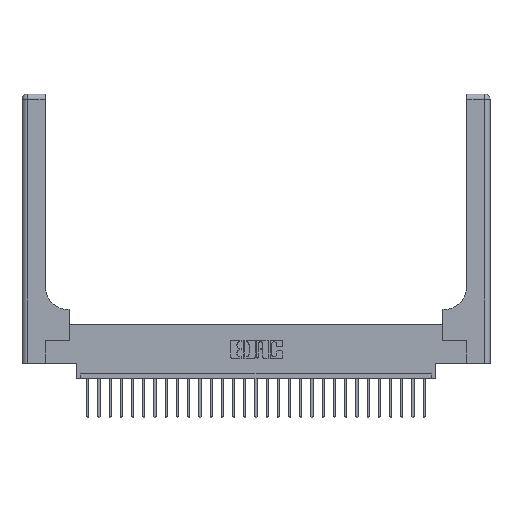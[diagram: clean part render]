
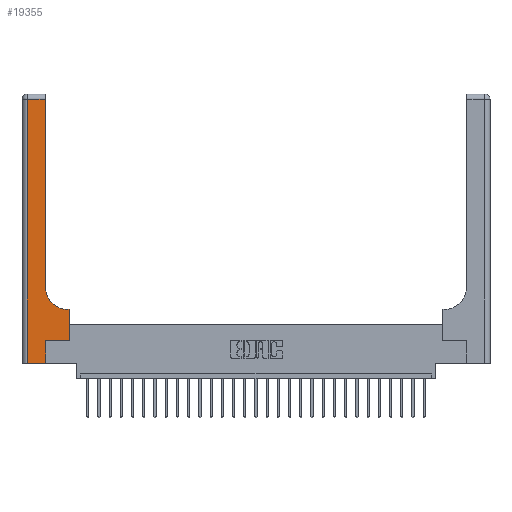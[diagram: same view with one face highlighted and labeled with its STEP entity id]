
A CAD part, top view. The second image highlights one B-rep face of the part: STEP entity #19355.
In plain terms, the highlighted planar face has unit normal (0, 0, 1).
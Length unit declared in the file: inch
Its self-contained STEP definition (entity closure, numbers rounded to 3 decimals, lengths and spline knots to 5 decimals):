
#160 = CARTESIAN_POINT ( 'NONE',  ( 0.06, 3., 0.37 ) ) ;
#386 = DIRECTION ( 'NONE',  ( 1., 0., 0. ) ) ;
#827 = CARTESIAN_POINT ( 'NONE',  ( 0.265, 0.25, 0.37 ) ) ;
#878 = CARTESIAN_POINT ( 'NONE',  ( 0., 0., 0.37 ) ) ;
#897 = EDGE_CURVE ( 'NONE', #14503, #10688, #25586, .T. ) ;
#1020 = PLANE ( 'NONE',  #8135 ) ;
#1361 = EDGE_CURVE ( 'NONE', #11129, #23837, #13041, .T. ) ;
#1598 = LINE ( 'NONE', #22780, #13895 ) ;
#1727 = EDGE_CURVE ( 'NONE', #13313, #22823, #15457, .T. ) ;
#2290 = CARTESIAN_POINT ( 'NONE',  ( 0.265, 0., 0.37 ) ) ;
#2490 = ORIENTED_EDGE ( 'NONE', *, *, #13686, .T. ) ;
#2798 = LINE ( 'NONE', #878, #13047 ) ;
#3026 = CARTESIAN_POINT ( 'NONE',  ( 0., 3., 0.37 ) ) ;
#3300 = VERTEX_POINT ( 'NONE', #10138 ) ;
#4204 = DIRECTION ( 'NONE',  ( 0., 1., 0. ) ) ;
#4282 = DIRECTION ( 'NONE',  ( 0., 1., 0. ) ) ;
#4557 = CARTESIAN_POINT ( 'NONE',  ( 0.51, 0.85, 0.37 ) ) ;
#4723 = DIRECTION ( 'NONE',  ( -1., 0., 0. ) ) ;
#4737 = ORIENTED_EDGE ( 'NONE', *, *, #11820, .T. ) ;
#5027 = DIRECTION ( 'NONE',  ( 0., 0., -1. ) ) ;
#5046 = LINE ( 'NONE', #19664, #20202 ) ;
#6188 = DIRECTION ( 'NONE',  ( 0., -1., 0. ) ) ;
#6428 = CARTESIAN_POINT ( 'NONE',  ( 0.528, 0.25, 0.37 ) ) ;
#6614 = AXIS2_PLACEMENT_3D ( 'NONE', #4557, #14737, #386 ) ;
#6826 = CARTESIAN_POINT ( 'NONE',  ( 0.528, 0.6, 0.37 ) ) ;
#6858 = VECTOR ( 'NONE', #12193, 39.37008 ) ;
#8135 = AXIS2_PLACEMENT_3D ( 'NONE', #3026, #5027, #19159 ) ;
#8582 = EDGE_LOOP ( 'NONE', ( #12353, #25006, #9893, #16631, #10606, #4737, #22381, #2490, #20142 ) ) ;
#8651 = VECTOR ( 'NONE', #4723, 39.37008 ) ;
#9507 = VECTOR ( 'NONE', #6188, 39.37008 ) ;
#9630 = EDGE_CURVE ( 'NONE', #23837, #3300, #1598, .T. ) ;
#9893 = ORIENTED_EDGE ( 'NONE', *, *, #897, .T. ) ;
#10138 = CARTESIAN_POINT ( 'NONE',  ( 0.26, 2.94, 0.37 ) ) ;
#10338 = CARTESIAN_POINT ( 'NONE',  ( 0.265, 0.25, 0.37 ) ) ;
#10366 = EDGE_CURVE ( 'NONE', #3300, #14503, #5046, .T. ) ;
#10606 = ORIENTED_EDGE ( 'NONE', *, *, #1727, .T. ) ;
#10688 = VERTEX_POINT ( 'NONE', #22925 ) ;
#11129 = VERTEX_POINT ( 'NONE', #23139 ) ;
#11820 = EDGE_CURVE ( 'NONE', #22823, #21023, #24253, .T. ) ;
#12193 = DIRECTION ( 'NONE',  ( 1., 0., 0. ) ) ;
#12239 = CARTESIAN_POINT ( 'NONE',  ( 0.06, 2.94, 0.37 ) ) ;
#12301 = EDGE_CURVE ( 'NONE', #21023, #16313, #16001, .T. ) ;
#12353 = ORIENTED_EDGE ( 'NONE', *, *, #9630, .T. ) ;
#13041 = CIRCLE ( 'NONE', #6614, 0.25 ) ;
#13047 = VECTOR ( 'NONE', #18924, 39.37008 ) ;
#13313 = VERTEX_POINT ( 'NONE', #20820 ) ;
#13686 = EDGE_CURVE ( 'NONE', #16313, #11129, #18451, .T. ) ;
#13774 = DIRECTION ( 'NONE',  ( -1., 0., 0. ) ) ;
#13895 = VECTOR ( 'NONE', #24835, 39.37008 ) ;
#14503 = VERTEX_POINT ( 'NONE', #12239 ) ;
#14737 = DIRECTION ( 'NONE',  ( 0., 0., -1. ) ) ;
#14898 = CARTESIAN_POINT ( 'NONE',  ( 0.26, 0.6, 0.37 ) ) ;
#15199 = EDGE_CURVE ( 'NONE', #10688, #13313, #2798, .T. ) ;
#15457 = LINE ( 'NONE', #2290, #24271 ) ;
#16001 = LINE ( 'NONE', #24309, #19163 ) ;
#16174 = CARTESIAN_POINT ( 'NONE',  ( 0.26, 0.85, 0.37 ) ) ;
#16313 = VERTEX_POINT ( 'NONE', #6826 ) ;
#16631 = ORIENTED_EDGE ( 'NONE', *, *, #15199, .T. ) ;
#18451 = LINE ( 'NONE', #14898, #8651 ) ;
#18924 = DIRECTION ( 'NONE',  ( 1., 0., 0. ) ) ;
#19159 = DIRECTION ( 'NONE',  ( -1., 0., 0. ) ) ;
#19163 = VECTOR ( 'NONE', #4282, 39.37008 ) ;
#19355 = ADVANCED_FACE ( 'NONE', ( #22119 ), #1020, .F. ) ;
#19664 = CARTESIAN_POINT ( 'NONE',  ( 0., 2.94, 0.37 ) ) ;
#20142 = ORIENTED_EDGE ( 'NONE', *, *, #1361, .T. ) ;
#20202 = VECTOR ( 'NONE', #13774, 39.37008 ) ;
#20820 = CARTESIAN_POINT ( 'NONE',  ( 0.265, 0., 0.37 ) ) ;
#21023 = VERTEX_POINT ( 'NONE', #6428 ) ;
#22119 = FACE_OUTER_BOUND ( 'NONE', #8582, .T. ) ;
#22381 = ORIENTED_EDGE ( 'NONE', *, *, #12301, .T. ) ;
#22780 = CARTESIAN_POINT ( 'NONE',  ( 0.26, 3., 0.37 ) ) ;
#22823 = VERTEX_POINT ( 'NONE', #827 ) ;
#22925 = CARTESIAN_POINT ( 'NONE',  ( 0.06, 0., 0.37 ) ) ;
#23139 = CARTESIAN_POINT ( 'NONE',  ( 0.51, 0.6, 0.37 ) ) ;
#23837 = VERTEX_POINT ( 'NONE', #16174 ) ;
#24253 = LINE ( 'NONE', #10338, #6858 ) ;
#24271 = VECTOR ( 'NONE', #4204, 39.37008 ) ;
#24309 = CARTESIAN_POINT ( 'NONE',  ( 0.528, 0.25, 0.37 ) ) ;
#24835 = DIRECTION ( 'NONE',  ( 0., 1., 0. ) ) ;
#25006 = ORIENTED_EDGE ( 'NONE', *, *, #10366, .T. ) ;
#25586 = LINE ( 'NONE', #160, #9507 ) ;
